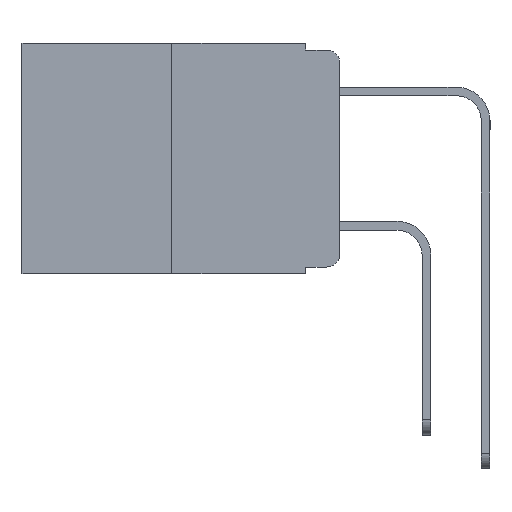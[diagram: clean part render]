
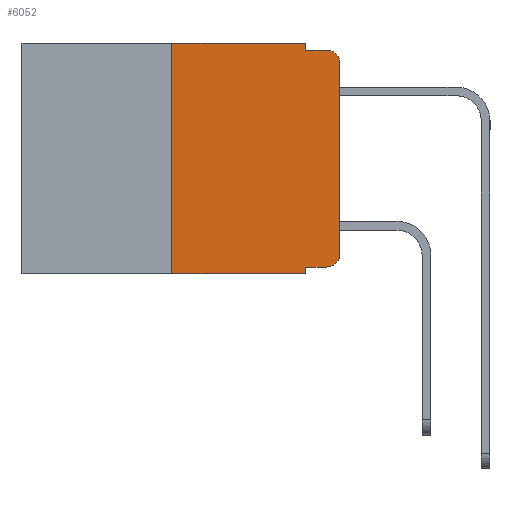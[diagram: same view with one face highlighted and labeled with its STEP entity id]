
A CAD part, left-side view. The second image highlights one B-rep face of the part: STEP entity #6052.
In plain terms, the highlighted planar face has unit normal (-1, 0, 0).
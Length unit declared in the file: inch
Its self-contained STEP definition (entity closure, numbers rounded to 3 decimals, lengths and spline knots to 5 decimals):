
#106 = LINE ( 'NONE', #760, #10421 ) ;
#379 = ORIENTED_EDGE ( 'NONE', *, *, #2896, .F. ) ;
#760 = CARTESIAN_POINT ( 'NONE',  ( 0., 0.473, -0.343 ) ) ;
#837 = VERTEX_POINT ( 'NONE', #6744 ) ;
#851 = FACE_OUTER_BOUND ( 'NONE', #1121, .T. ) ;
#870 = CARTESIAN_POINT ( 'NONE',  ( 0., 0.25, 0. ) ) ;
#963 = CARTESIAN_POINT ( 'NONE',  ( 0., 0.051, -0.333 ) ) ;
#1121 = EDGE_LOOP ( 'NONE', ( #4976, #1835, #10688, #11443, #11630, #6856, #4997, #379, #5420, #8068 ) ) ;
#1157 = AXIS2_PLACEMENT_3D ( 'NONE', #12457, #12505, #11358 ) ;
#1182 = CARTESIAN_POINT ( 'NONE',  ( 0., 0.051, -0.333 ) ) ;
#1290 = EDGE_CURVE ( 'NONE', #3395, #8852, #2235, .T. ) ;
#1444 = CARTESIAN_POINT ( 'NONE',  ( 0., 0., -0.03 ) ) ;
#1835 = ORIENTED_EDGE ( 'NONE', *, *, #12283, .T. ) ;
#1861 = DIRECTION ( 'NONE',  ( 0., -1., 0. ) ) ;
#1934 = CARTESIAN_POINT ( 'NONE',  ( 0., 0.473, 0. ) ) ;
#2182 = LINE ( 'NONE', #5988, #12403 ) ;
#2235 = CIRCLE ( 'NONE', #1157, 0.02 ) ;
#2729 = EDGE_CURVE ( 'NONE', #4758, #10298, #6618, .T. ) ;
#2778 = CARTESIAN_POINT ( 'NONE',  ( 0., 0.051, 0. ) ) ;
#2822 = VECTOR ( 'NONE', #12749, 39.37008 ) ;
#2872 = CARTESIAN_POINT ( 'NONE',  ( 0., 0.473, 0. ) ) ;
#2896 = EDGE_CURVE ( 'NONE', #11382, #837, #7391, .T. ) ;
#2956 = DIRECTION ( 'NONE',  ( 1., 0., 0. ) ) ;
#2976 = CIRCLE ( 'NONE', #12855, 0.02 ) ;
#3395 = VERTEX_POINT ( 'NONE', #4638 ) ;
#3561 = EDGE_CURVE ( 'NONE', #9302, #837, #106, .T. ) ;
#3810 = LINE ( 'NONE', #870, #2822 ) ;
#4140 = DIRECTION ( 'NONE',  ( 0., 0., -1. ) ) ;
#4398 = CARTESIAN_POINT ( 'NONE',  ( 0., 0.25, -0.343 ) ) ;
#4415 = LINE ( 'NONE', #6131, #9670 ) ;
#4517 = VERTEX_POINT ( 'NONE', #7344 ) ;
#4630 = DIRECTION ( 'NONE',  ( -1., 0., 0. ) ) ;
#4638 = CARTESIAN_POINT ( 'NONE',  ( 0., 0.02, -0.333 ) ) ;
#4686 = AXIS2_PLACEMENT_3D ( 'NONE', #1934, #2956, #9908 ) ;
#4758 = VERTEX_POINT ( 'NONE', #10621 ) ;
#4851 = DIRECTION ( 'NONE',  ( 0., -1., 0. ) ) ;
#4936 = CARTESIAN_POINT ( 'NONE',  ( 0., 0.25, 0. ) ) ;
#4976 = ORIENTED_EDGE ( 'NONE', *, *, #10243, .T. ) ;
#4997 = ORIENTED_EDGE ( 'NONE', *, *, #3561, .T. ) ;
#5366 = VERTEX_POINT ( 'NONE', #4936 ) ;
#5420 = ORIENTED_EDGE ( 'NONE', *, *, #11519, .T. ) ;
#5988 = CARTESIAN_POINT ( 'NONE',  ( 0., 0., 0. ) ) ;
#6052 = ADVANCED_FACE ( 'NONE', ( #851 ), #7928, .F. ) ;
#6131 = CARTESIAN_POINT ( 'NONE',  ( 0., 0.051, 0. ) ) ;
#6500 = CARTESIAN_POINT ( 'NONE',  ( 0., 0., -0.313 ) ) ;
#6618 = LINE ( 'NONE', #8446, #9227 ) ;
#6744 = CARTESIAN_POINT ( 'NONE',  ( 0., 0.051, -0.343 ) ) ;
#6856 = ORIENTED_EDGE ( 'NONE', *, *, #10175, .F. ) ;
#7081 = CARTESIAN_POINT ( 'NONE',  ( 0., 0.02, -0.01 ) ) ;
#7344 = CARTESIAN_POINT ( 'NONE',  ( 0., 0.051, 0. ) ) ;
#7391 = LINE ( 'NONE', #2778, #12273 ) ;
#7928 = PLANE ( 'NONE',  #4686 ) ;
#8068 = ORIENTED_EDGE ( 'NONE', *, *, #1290, .T. ) ;
#8177 = DIRECTION ( 'NONE',  ( 0., -1., 0. ) ) ;
#8446 = CARTESIAN_POINT ( 'NONE',  ( 0., 0.051, -0.01 ) ) ;
#8852 = VERTEX_POINT ( 'NONE', #6500 ) ;
#8896 = VERTEX_POINT ( 'NONE', #1444 ) ;
#9227 = VECTOR ( 'NONE', #12417, 39.37008 ) ;
#9302 = VERTEX_POINT ( 'NONE', #4398 ) ;
#9530 = VECTOR ( 'NONE', #1861, 39.37008 ) ;
#9670 = VECTOR ( 'NONE', #4140, 39.37008 ) ;
#9847 = LINE ( 'NONE', #2872, #9530 ) ;
#9908 = DIRECTION ( 'NONE',  ( 0., 0., -1. ) ) ;
#10175 = EDGE_CURVE ( 'NONE', #9302, #5366, #3810, .T. ) ;
#10243 = EDGE_CURVE ( 'NONE', #8852, #8896, #2182, .T. ) ;
#10298 = VERTEX_POINT ( 'NONE', #7081 ) ;
#10421 = VECTOR ( 'NONE', #4851, 39.37008 ) ;
#10519 = CARTESIAN_POINT ( 'NONE',  ( 0., 0.02, -0.03 ) ) ;
#10621 = CARTESIAN_POINT ( 'NONE',  ( 0., 0.051, -0.01 ) ) ;
#10688 = ORIENTED_EDGE ( 'NONE', *, *, #2729, .F. ) ;
#10707 = DIRECTION ( 'NONE',  ( 0., 0., -1. ) ) ;
#10926 = DIRECTION ( 'NONE',  ( 0., 0., 1. ) ) ;
#11283 = EDGE_CURVE ( 'NONE', #5366, #4517, #9847, .T. ) ;
#11358 = DIRECTION ( 'NONE',  ( 0., 0., -1. ) ) ;
#11382 = VERTEX_POINT ( 'NONE', #963 ) ;
#11443 = ORIENTED_EDGE ( 'NONE', *, *, #12606, .F. ) ;
#11499 = DIRECTION ( 'NONE',  ( 0., 0., -1. ) ) ;
#11519 = EDGE_CURVE ( 'NONE', #11382, #3395, #12272, .T. ) ;
#11630 = ORIENTED_EDGE ( 'NONE', *, *, #11283, .F. ) ;
#11955 = VECTOR ( 'NONE', #8177, 39.37008 ) ;
#12272 = LINE ( 'NONE', #1182, #11955 ) ;
#12273 = VECTOR ( 'NONE', #10707, 39.37008 ) ;
#12283 = EDGE_CURVE ( 'NONE', #8896, #10298, #2976, .T. ) ;
#12403 = VECTOR ( 'NONE', #10926, 39.37008 ) ;
#12417 = DIRECTION ( 'NONE',  ( 0., -1., 0. ) ) ;
#12457 = CARTESIAN_POINT ( 'NONE',  ( 0., 0.02, -0.313 ) ) ;
#12505 = DIRECTION ( 'NONE',  ( -1., 0., 0. ) ) ;
#12606 = EDGE_CURVE ( 'NONE', #4517, #4758, #4415, .T. ) ;
#12749 = DIRECTION ( 'NONE',  ( 0., 0., 1. ) ) ;
#12855 = AXIS2_PLACEMENT_3D ( 'NONE', #10519, #4630, #11499 ) ;
